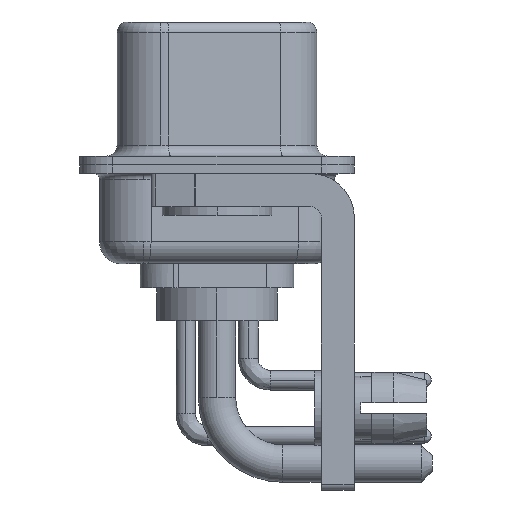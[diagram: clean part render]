
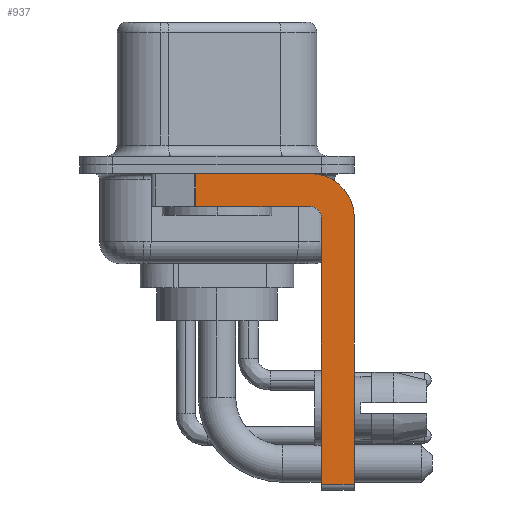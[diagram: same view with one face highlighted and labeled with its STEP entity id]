
A CAD part, left-side view. The second image highlights one B-rep face of the part: STEP entity #937.
In plain terms, the highlighted planar face has unit normal (-1, 0, 0).
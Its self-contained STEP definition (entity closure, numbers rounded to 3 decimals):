
#40 = EDGE_CURVE ( 'NONE', #1677, #11358, #3860, .T. ) ;
#312 = DIRECTION ( 'NONE',  ( 0., 0., 1. ) ) ;
#695 = CIRCLE ( 'NONE', #19116, 0.5 ) ;
#718 = DIRECTION ( 'NONE',  ( 0., 0., -1. ) ) ;
#735 = ORIENTED_EDGE ( 'NONE', *, *, #5876, .T. ) ;
#847 = CIRCLE ( 'NONE', #3868, 2. ) ;
#937 = ADVANCED_FACE ( 'NONE', ( #3912 ), #4258, .F. ) ;
#950 = CARTESIAN_POINT ( 'NONE',  ( -2.9, -4.25, -1.9 ) ) ;
#1512 = DIRECTION ( 'NONE',  ( -1., 0., 0. ) ) ;
#1677 = VERTEX_POINT ( 'NONE', #5410 ) ;
#2025 = DIRECTION ( 'NONE',  ( 0., 0., -1. ) ) ;
#2496 = VECTOR ( 'NONE', #312, 1000. ) ;
#3666 = EDGE_CURVE ( 'NONE', #21956, #18600, #847, .T. ) ;
#3678 = DIRECTION ( 'NONE',  ( 0., -1., 0. ) ) ;
#3860 = LINE ( 'NONE', #16452, #2496 ) ;
#3868 = AXIS2_PLACEMENT_3D ( 'NONE', #5787, #18166, #2025 ) ;
#3912 = FACE_OUTER_BOUND ( 'NONE', #4235, .T. ) ;
#3979 = VERTEX_POINT ( 'NONE', #17062 ) ;
#4190 = CARTESIAN_POINT ( 'NONE',  ( -2.9, 0.978, -0.4 ) ) ;
#4235 = EDGE_LOOP ( 'NONE', ( #11787, #8293, #23006, #15301, #23271, #735, #22048, #9825 ) ) ;
#4258 = PLANE ( 'NONE',  #19197 ) ;
#5410 = CARTESIAN_POINT ( 'NONE',  ( -2.9, -4.75, -14.55 ) ) ;
#5785 = DIRECTION ( 'NONE',  ( 1., 0., 0. ) ) ;
#5787 = CARTESIAN_POINT ( 'NONE',  ( -2.9, -4.25, -2.4 ) ) ;
#5876 = EDGE_CURVE ( 'NONE', #1677, #3979, #20278, .T. ) ;
#6761 = CARTESIAN_POINT ( 'NONE',  ( -2.9, 0.978, -1.9 ) ) ;
#7260 = DIRECTION ( 'NONE',  ( 0., 0., -1. ) ) ;
#7658 = CARTESIAN_POINT ( 'NONE',  ( -2.9, -6.25, -2.4 ) ) ;
#8293 = ORIENTED_EDGE ( 'NONE', *, *, #10554, .T. ) ;
#8298 = LINE ( 'NONE', #17112, #17997 ) ;
#8987 = CARTESIAN_POINT ( 'NONE',  ( -2.9, -6.25, -2.4 ) ) ;
#9663 = CARTESIAN_POINT ( 'NONE',  ( -2.9, -4.25, -2.4 ) ) ;
#9771 = DIRECTION ( 'NONE',  ( 0., -1., 0. ) ) ;
#9825 = ORIENTED_EDGE ( 'NONE', *, *, #3666, .F. ) ;
#10554 = EDGE_CURVE ( 'NONE', #13955, #12316, #14204, .T. ) ;
#11313 = CARTESIAN_POINT ( 'NONE',  ( -2.9, -4.25, -14.55 ) ) ;
#11358 = VERTEX_POINT ( 'NONE', #14380 ) ;
#11787 = ORIENTED_EDGE ( 'NONE', *, *, #19849, .F. ) ;
#12022 = EDGE_CURVE ( 'NONE', #11358, #17925, #695, .T. ) ;
#12154 = EDGE_CURVE ( 'NONE', #17925, #12316, #8298, .T. ) ;
#12316 = VERTEX_POINT ( 'NONE', #6761 ) ;
#12894 = CARTESIAN_POINT ( 'NONE',  ( -2.9, 0.978, -1.9 ) ) ;
#13692 = DIRECTION ( 'NONE',  ( 0., 1., 0. ) ) ;
#13955 = VERTEX_POINT ( 'NONE', #4190 ) ;
#14150 = VECTOR ( 'NONE', #7260, 1000. ) ;
#14204 = LINE ( 'NONE', #12894, #14150 ) ;
#14376 = CARTESIAN_POINT ( 'NONE',  ( -2.9, 3., -0.4 ) ) ;
#14380 = CARTESIAN_POINT ( 'NONE',  ( -2.9, -4.75, -2.4 ) ) ;
#14491 = DIRECTION ( 'NONE',  ( 0., 0., -1. ) ) ;
#14731 = LINE ( 'NONE', #14376, #21398 ) ;
#15301 = ORIENTED_EDGE ( 'NONE', *, *, #12022, .F. ) ;
#15629 = CARTESIAN_POINT ( 'NONE',  ( -2.9, -4.25, -2.4 ) ) ;
#15748 = DIRECTION ( 'NONE',  ( 0., 0., 1. ) ) ;
#16021 = CARTESIAN_POINT ( 'NONE',  ( -2.9, -4.25, -0.4 ) ) ;
#16452 = CARTESIAN_POINT ( 'NONE',  ( -2.9, -4.75, -14.8 ) ) ;
#17062 = CARTESIAN_POINT ( 'NONE',  ( -2.9, -6.25, -14.55 ) ) ;
#17112 = CARTESIAN_POINT ( 'NONE',  ( -2.9, -4.25, -1.9 ) ) ;
#17925 = VERTEX_POINT ( 'NONE', #950 ) ;
#17997 = VECTOR ( 'NONE', #13692, 1000. ) ;
#18166 = DIRECTION ( 'NONE',  ( 1., 0., 0. ) ) ;
#18371 = VECTOR ( 'NONE', #14491, 1000. ) ;
#18600 = VERTEX_POINT ( 'NONE', #8987 ) ;
#19116 = AXIS2_PLACEMENT_3D ( 'NONE', #15629, #1512, #15748 ) ;
#19197 = AXIS2_PLACEMENT_3D ( 'NONE', #9663, #5785, #718 ) ;
#19849 = EDGE_CURVE ( 'NONE', #13955, #21956, #14731, .T. ) ;
#19904 = EDGE_CURVE ( 'NONE', #18600, #3979, #22052, .T. ) ;
#20278 = LINE ( 'NONE', #11313, #22322 ) ;
#21398 = VECTOR ( 'NONE', #3678, 1000. ) ;
#21956 = VERTEX_POINT ( 'NONE', #16021 ) ;
#22048 = ORIENTED_EDGE ( 'NONE', *, *, #19904, .F. ) ;
#22052 = LINE ( 'NONE', #7658, #18371 ) ;
#22322 = VECTOR ( 'NONE', #9771, 1000. ) ;
#23006 = ORIENTED_EDGE ( 'NONE', *, *, #12154, .F. ) ;
#23271 = ORIENTED_EDGE ( 'NONE', *, *, #40, .F. ) ;
